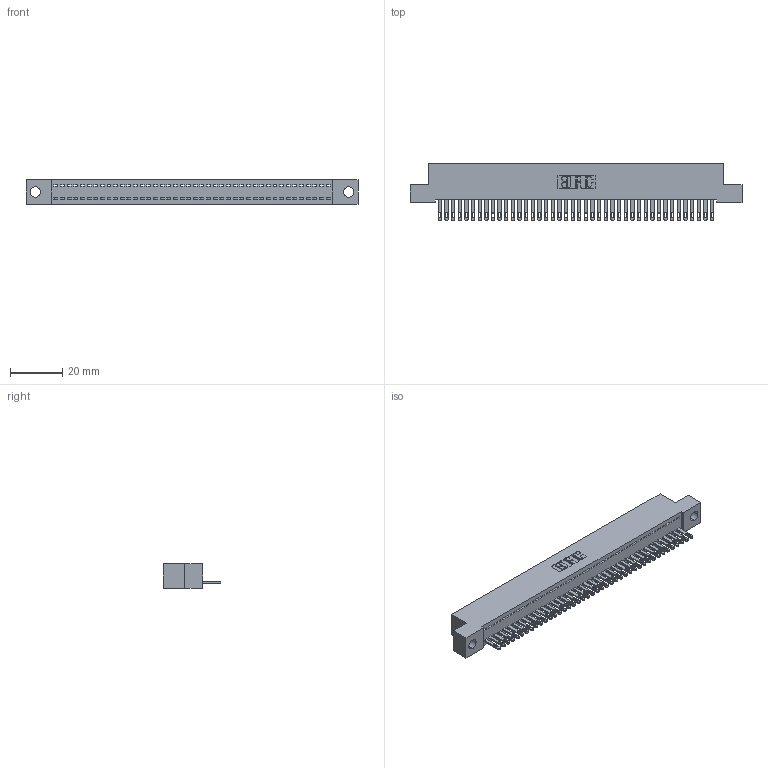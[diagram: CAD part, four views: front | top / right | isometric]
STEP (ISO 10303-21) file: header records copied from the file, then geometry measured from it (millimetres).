
FILE_DESCRIPTION (( 'STEP AP203' ), '1' );
FILE_NAME ('342-042-500-104.STEP', '2018-08-12T02:05:13', ( '' ), ( '' ), 'SwSTEP 2.0', 'SolidWorks 2016', '' );
FILE_SCHEMA (( 'CONFIG_CONTROL_DESIGN' ));
Length unit declared in the file: inch
Products named in the file (3): 345-292-001_345-293-100; 342-042-500-104; 342 Part_.156 TH
Assembly tree (43 placements, depth 2):
  342-042-500-104
    342 Part_.156 TH
    345-292-001_345-293-100  x42
Bounding box: 127 x 21.85 x 9.4 mm (x, y, z)
Volume: 11074.3 mm3; surface area: 16163.6 mm2
Topology: 43 solids, 43 shells, 2378 faces, 7355 edges, 4902 vertices
Faces by surface type: plane 1578, cylinder 800
Entity records: 25477 total; most frequent: CARTESIAN_POINT 4400, ORIENTED_EDGE 4378, DIRECTION 3713, EDGE_CURVE 2189, LINE 2057, VECTOR 2057, VERTEX_POINT 1458, AXIS2_PLACEMENT_3D 828
